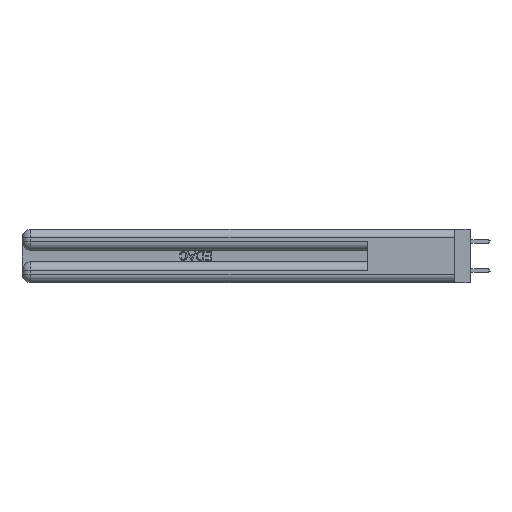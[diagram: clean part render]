
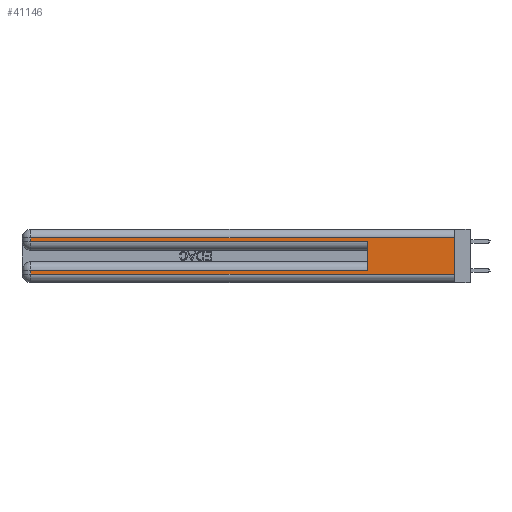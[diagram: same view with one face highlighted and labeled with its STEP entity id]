
A CAD part, left-side view. The second image highlights one B-rep face of the part: STEP entity #41146.
In plain terms, the highlighted planar face has unit normal (-1, 0, 0).
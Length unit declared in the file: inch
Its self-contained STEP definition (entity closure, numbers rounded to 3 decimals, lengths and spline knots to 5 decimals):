
#61 = EDGE_CURVE ( 'NONE', #1097, #19594, #43275, .T. ) ;
#1064 = CARTESIAN_POINT ( 'NONE',  ( 0., 0., 0.06 ) ) ;
#1097 = VERTEX_POINT ( 'NONE', #41856 ) ;
#1309 = VERTEX_POINT ( 'NONE', #6433 ) ;
#1474 = ORIENTED_EDGE ( 'NONE', *, *, #18060, .T. ) ;
#2433 = LINE ( 'NONE', #11008, #2954 ) ;
#2477 = CARTESIAN_POINT ( 'NONE',  ( 0., 0., 0.31 ) ) ;
#2954 = VECTOR ( 'NONE', #32204, 39.37008 ) ;
#3768 = VERTEX_POINT ( 'NONE', #32655 ) ;
#5817 = DIRECTION ( 'NONE',  ( 0., 1., 0. ) ) ;
#6250 = DIRECTION ( 'NONE',  ( 0., 1., 0. ) ) ;
#6433 = CARTESIAN_POINT ( 'NONE',  ( 0., 0.6, 0.085 ) ) ;
#7428 = ORIENTED_EDGE ( 'NONE', *, *, #16276, .T. ) ;
#8250 = CARTESIAN_POINT ( 'NONE',  ( 0., 2.94, 0.285 ) ) ;
#8842 = CARTESIAN_POINT ( 'NONE',  ( 0., 0., 0.285 ) ) ;
#8911 = VERTEX_POINT ( 'NONE', #8250 ) ;
#9834 = CARTESIAN_POINT ( 'NONE',  ( 0., 0., 0.37 ) ) ;
#9922 = FACE_OUTER_BOUND ( 'NONE', #23227, .T. ) ;
#10506 = CARTESIAN_POINT ( 'NONE',  ( 0., 0., 0.06 ) ) ;
#11008 = CARTESIAN_POINT ( 'NONE',  ( 0., 2.94, 0.37 ) ) ;
#11824 = CARTESIAN_POINT ( 'NONE',  ( 0., 0., 0.37 ) ) ;
#12740 = ORIENTED_EDGE ( 'NONE', *, *, #36092, .F. ) ;
#13173 = VECTOR ( 'NONE', #17146, 39.37008 ) ;
#13447 = DIRECTION ( 'NONE',  ( 0., 0., -1. ) ) ;
#13526 = VECTOR ( 'NONE', #39010, 39.37008 ) ;
#14223 = ORIENTED_EDGE ( 'NONE', *, *, #23565, .T. ) ;
#15167 = DIRECTION ( 'NONE',  ( 0., 0., -1. ) ) ;
#16276 = EDGE_CURVE ( 'NONE', #8911, #43496, #38827, .T. ) ;
#17056 = VECTOR ( 'NONE', #6250, 39.37008 ) ;
#17146 = DIRECTION ( 'NONE',  ( 0., -1., 0. ) ) ;
#17572 = AXIS2_PLACEMENT_3D ( 'NONE', #11824, #32114, #15167 ) ;
#18060 = EDGE_CURVE ( 'NONE', #27532, #3768, #27376, .T. ) ;
#18882 = LINE ( 'NONE', #42497, #13526 ) ;
#18984 = DIRECTION ( 'NONE',  ( 0., -1., 0. ) ) ;
#19594 = VERTEX_POINT ( 'NONE', #1064 ) ;
#19994 = CARTESIAN_POINT ( 'NONE',  ( 0., 0., 0.085 ) ) ;
#20425 = VECTOR ( 'NONE', #18984, 39.37008 ) ;
#21440 = EDGE_CURVE ( 'NONE', #1309, #43496, #43721, .T. ) ;
#21593 = ORIENTED_EDGE ( 'NONE', *, *, #43322, .T. ) ;
#23227 = EDGE_LOOP ( 'NONE', ( #12740, #1474, #14223, #7428, #39112, #36471, #21593, #25053 ) ) ;
#23565 = EDGE_CURVE ( 'NONE', #3768, #8911, #2433, .T. ) ;
#25053 = ORIENTED_EDGE ( 'NONE', *, *, #61, .T. ) ;
#27376 = LINE ( 'NONE', #44810, #17056 ) ;
#27532 = VERTEX_POINT ( 'NONE', #2477 ) ;
#28589 = CARTESIAN_POINT ( 'NONE',  ( 0., 2.94, 0.085 ) ) ;
#31276 = LINE ( 'NONE', #9834, #36098 ) ;
#32114 = DIRECTION ( 'NONE',  ( 1., 0., 0. ) ) ;
#32204 = DIRECTION ( 'NONE',  ( 0., 0., -1. ) ) ;
#32655 = CARTESIAN_POINT ( 'NONE',  ( 0., 2.94, 0.31 ) ) ;
#33420 = CARTESIAN_POINT ( 'NONE',  ( 0., 0.6, 0.285 ) ) ;
#34440 = VERTEX_POINT ( 'NONE', #28589 ) ;
#35367 = EDGE_CURVE ( 'NONE', #1309, #34440, #39408, .T. ) ;
#35574 = VECTOR ( 'NONE', #35994, 39.37008 ) ;
#35605 = VECTOR ( 'NONE', #5817, 39.37008 ) ;
#35994 = DIRECTION ( 'NONE',  ( 0., 0., 1. ) ) ;
#36092 = EDGE_CURVE ( 'NONE', #27532, #19594, #31276, .T. ) ;
#36098 = VECTOR ( 'NONE', #13447, 39.37008 ) ;
#36170 = PLANE ( 'NONE',  #17572 ) ;
#36471 = ORIENTED_EDGE ( 'NONE', *, *, #35367, .T. ) ;
#38827 = LINE ( 'NONE', #8842, #20425 ) ;
#39010 = DIRECTION ( 'NONE',  ( 0., 0., -1. ) ) ;
#39112 = ORIENTED_EDGE ( 'NONE', *, *, #21440, .F. ) ;
#39323 = CARTESIAN_POINT ( 'NONE',  ( 0., 0.6, 0.145 ) ) ;
#39408 = LINE ( 'NONE', #19994, #35605 ) ;
#41146 = ADVANCED_FACE ( 'NONE', ( #9922 ), #36170, .F. ) ;
#41856 = CARTESIAN_POINT ( 'NONE',  ( 0., 2.94, 0.06 ) ) ;
#42497 = CARTESIAN_POINT ( 'NONE',  ( 0., 2.94, 0.37 ) ) ;
#43275 = LINE ( 'NONE', #10506, #13173 ) ;
#43322 = EDGE_CURVE ( 'NONE', #34440, #1097, #18882, .T. ) ;
#43496 = VERTEX_POINT ( 'NONE', #33420 ) ;
#43721 = LINE ( 'NONE', #39323, #35574 ) ;
#44810 = CARTESIAN_POINT ( 'NONE',  ( 0., 0., 0.31 ) ) ;
